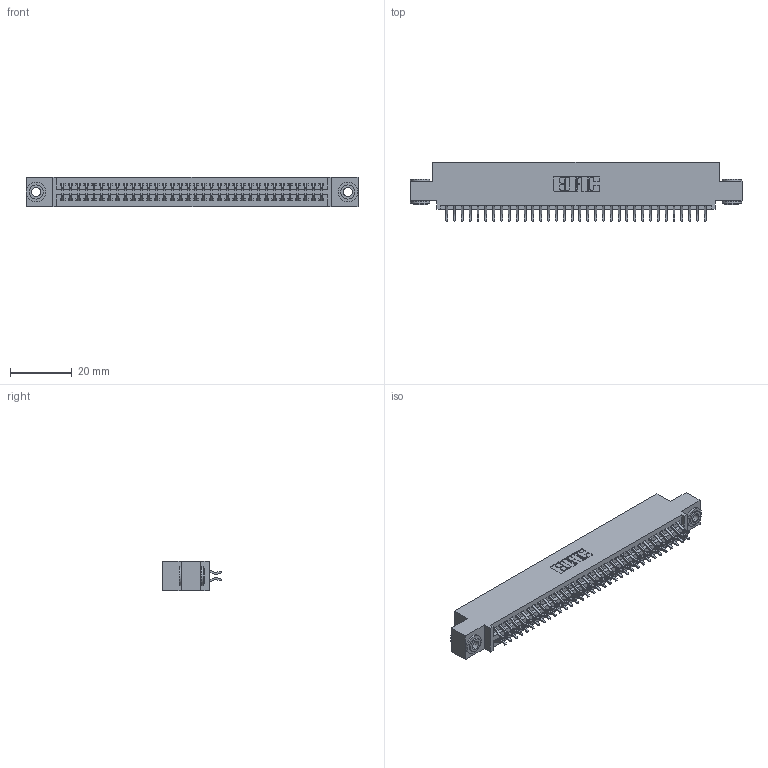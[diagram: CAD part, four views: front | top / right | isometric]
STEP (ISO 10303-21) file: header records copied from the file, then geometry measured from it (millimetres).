
FILE_DESCRIPTION (( 'STEP AP203' ), '1' );
FILE_NAME ('395-068-556-503.STEP', '2018-11-25T18:59:24', ( '' ), ( '' ), 'SwSTEP 2.0', 'SolidWorks 2016', '' );
FILE_SCHEMA (( 'CONFIG_CONTROL_DESIGN' ));
Length unit declared in the file: inch
Products named in the file (4): 345-250-002_345-250-002-102; 345-292-001_556 Tail; 345 Part_0.110 Offset - 0.156 Dia-TH; 395-068-556-503
Assembly tree (71 placements, depth 2):
  395-068-556-503
    345 Part_0.110 Offset - 0.156 Dia-TH
    345-292-001_556 Tail  x68
    345-250-002_345-250-002-102  x2
Bounding box: 107.57 x 19.24 x 9.4 mm (x, y, z)
Volume: 10318.4 mm3; surface area: 15335.6 mm2
Topology: 71 solids, 71 shells, 3976 faces, 11785 edges, 7762 vertices
Faces by surface type: plane 2610, cylinder 1358, cone 8
Entity records: 28756 total; most frequent: CARTESIAN_POINT 4819, ORIENTED_EDGE 4734, DIRECTION 4277, EDGE_CURVE 2367, LINE 2067, VECTOR 2067, VERTEX_POINT 1574, AXIS2_PLACEMENT_3D 1105
